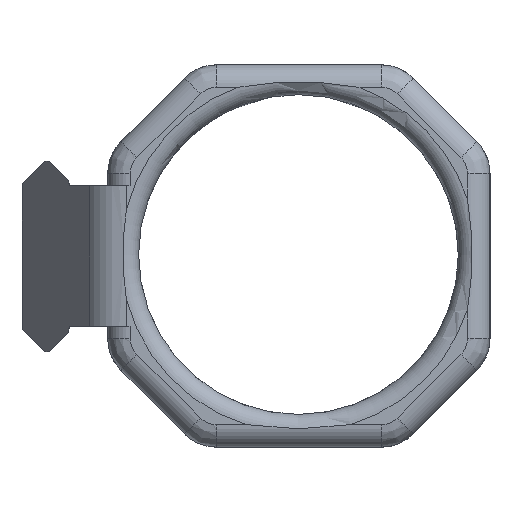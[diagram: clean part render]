
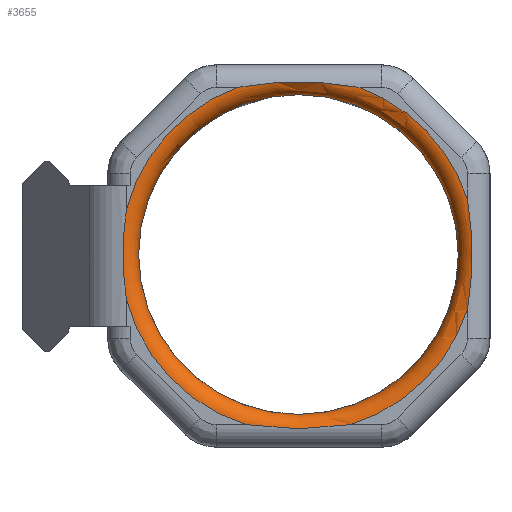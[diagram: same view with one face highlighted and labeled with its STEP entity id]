
A CAD part, left-side view. The second image highlights one B-rep face of the part: STEP entity #3655.
In plain terms, the highlighted toroidal (fillet/blend) face has major radius 19.771 mm and minor radius 2 mm.
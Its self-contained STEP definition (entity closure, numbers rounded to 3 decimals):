
#65=TOROIDAL_SURFACE('',#3895,19.771,2.);
#71=B_SPLINE_CURVE_WITH_KNOTS('',3,(#5442,#5443,#5444,#5445,#5446,#5447),
 .UNSPECIFIED.,.F.,.F.,(4,2,4),(0.498,0.996,0.998),
 .UNSPECIFIED.);
#72=B_SPLINE_CURVE_WITH_KNOTS('',3,(#5451,#5452,#5453,#5454,#5455,#5456,
#5457,#5458,#5459,#5460),.UNSPECIFIED.,.F.,.F.,(4,2,2,2,4),(-0.002,
0.,0.53,1.061,1.063),.UNSPECIFIED.);
#73=B_SPLINE_CURVE_WITH_KNOTS('',3,(#5464,#5465,#5466,#5467,#5468,#5469,
#5470,#5471,#5472,#5473),.UNSPECIFIED.,.F.,.F.,(4,2,2,2,4),(-0.002,
0.,0.584,1.169,1.171),.UNSPECIFIED.);
#74=B_SPLINE_CURVE_WITH_KNOTS('',3,(#5477,#5478,#5479,#5480,#5481,#5482,
#5483,#5484,#5485,#5486),.UNSPECIFIED.,.F.,.F.,(4,2,2,2,4),(-0.003,
0.,0.495,0.991,0.994),.UNSPECIFIED.);
#75=B_SPLINE_CURVE_WITH_KNOTS('',3,(#5489,#5490,#5491,#5492,#5493,#5494),
 .UNSPECIFIED.,.F.,.F.,(4,2,4),(-0.002,0.,0.498),
 .UNSPECIFIED.);
#286=FACE_OUTER_BOUND('',#485,.T.);
#485=EDGE_LOOP('',(#2614,#2615,#2616,#2617,#2618,#2619,#2620,#2621,#2622,
#2623,#2624,#2625,#2626));
#1461=CIRCLE('',#3896,17.771);
#1462=CIRCLE('',#3897,2.);
#1463=CIRCLE('',#3898,19.771);
#1464=CIRCLE('',#3899,19.771);
#1465=CIRCLE('',#3900,19.771);
#1466=CIRCLE('',#3901,19.771);
#1467=CIRCLE('',#3902,17.771);
#1619=VERTEX_POINT('',#5436);
#1620=VERTEX_POINT('',#5437);
#1621=VERTEX_POINT('',#5439);
#1622=VERTEX_POINT('',#5441);
#1623=VERTEX_POINT('',#5448);
#1624=VERTEX_POINT('',#5450);
#1625=VERTEX_POINT('',#5461);
#1626=VERTEX_POINT('',#5463);
#1627=VERTEX_POINT('',#5474);
#1628=VERTEX_POINT('',#5476);
#1629=VERTEX_POINT('',#5487);
#1999=EDGE_CURVE('',#1619,#1620,#1461,.T.);
#2000=EDGE_CURVE('',#1620,#1621,#1462,.T.);
#2001=EDGE_CURVE('',#1621,#1622,#71,.T.);
#2002=EDGE_CURVE('',#1622,#1623,#1463,.T.);
#2003=EDGE_CURVE('',#1623,#1624,#72,.T.);
#2004=EDGE_CURVE('',#1624,#1625,#1464,.T.);
#2005=EDGE_CURVE('',#1625,#1626,#73,.T.);
#2006=EDGE_CURVE('',#1626,#1627,#1465,.T.);
#2007=EDGE_CURVE('',#1627,#1628,#74,.T.);
#2008=EDGE_CURVE('',#1628,#1629,#1466,.T.);
#2009=EDGE_CURVE('',#1629,#1621,#75,.T.);
#2010=EDGE_CURVE('',#1620,#1619,#1467,.T.);
#2614=ORIENTED_EDGE('',*,*,#1999,.T.);
#2615=ORIENTED_EDGE('',*,*,#2000,.T.);
#2616=ORIENTED_EDGE('',*,*,#2001,.T.);
#2617=ORIENTED_EDGE('',*,*,#2002,.T.);
#2618=ORIENTED_EDGE('',*,*,#2003,.T.);
#2619=ORIENTED_EDGE('',*,*,#2004,.T.);
#2620=ORIENTED_EDGE('',*,*,#2005,.T.);
#2621=ORIENTED_EDGE('',*,*,#2006,.T.);
#2622=ORIENTED_EDGE('',*,*,#2007,.T.);
#2623=ORIENTED_EDGE('',*,*,#2008,.T.);
#2624=ORIENTED_EDGE('',*,*,#2009,.T.);
#2625=ORIENTED_EDGE('',*,*,#2000,.F.);
#2626=ORIENTED_EDGE('',*,*,#2010,.T.);
#3655=ADVANCED_FACE('',(#286),#65,.T.);
#3895=AXIS2_PLACEMENT_3D('',#5435,#4336,#4337);
#3896=AXIS2_PLACEMENT_3D('',#5438,#4338,#4339);
#3897=AXIS2_PLACEMENT_3D('',#5440,#4340,#4341);
#3898=AXIS2_PLACEMENT_3D('',#5449,#4342,#4343);
#3899=AXIS2_PLACEMENT_3D('',#5462,#4344,#4345);
#3900=AXIS2_PLACEMENT_3D('',#5475,#4346,#4347);
#3901=AXIS2_PLACEMENT_3D('',#5488,#4348,#4349);
#3902=AXIS2_PLACEMENT_3D('',#5495,#4350,#4351);
#4336=DIRECTION('center_axis',(-1.,0.,0.));
#4337=DIRECTION('ref_axis',(0.,0.,1.));
#4338=DIRECTION('center_axis',(1.,0.,0.));
#4339=DIRECTION('ref_axis',(0.,-1.,0.));
#4340=DIRECTION('center_axis',(0.,-1.,0.));
#4341=DIRECTION('ref_axis',(0.,0.,-1.));
#4342=DIRECTION('center_axis',(-1.,0.,0.));
#4343=DIRECTION('ref_axis',(0.,-1.,0.));
#4344=DIRECTION('center_axis',(-1.,0.,0.));
#4345=DIRECTION('ref_axis',(0.,-1.,0.));
#4346=DIRECTION('center_axis',(-1.,0.,0.));
#4347=DIRECTION('ref_axis',(0.,-1.,0.));
#4348=DIRECTION('center_axis',(-1.,0.,0.));
#4349=DIRECTION('ref_axis',(0.,-1.,0.));
#4350=DIRECTION('center_axis',(1.,0.,0.));
#4351=DIRECTION('ref_axis',(0.,-1.,0.));
#5435=CARTESIAN_POINT('Origin',(154.494,184.064,13.948));
#5436=CARTESIAN_POINT('',(154.494,201.835,13.948));
#5437=CARTESIAN_POINT('',(154.494,184.064,-3.823));
#5438=CARTESIAN_POINT('Origin',(154.494,184.064,13.948));
#5439=CARTESIAN_POINT('',(152.536,184.064,-5.416));
#5440=CARTESIAN_POINT('Origin',(154.494,184.064,-5.823));
#5441=CARTESIAN_POINT('',(152.494,178.29,-4.961));
#5442=CARTESIAN_POINT('Ctrl Pts',(152.536,184.064,-5.416));
#5443=CARTESIAN_POINT('Ctrl Pts',(152.536,181.868,-5.416));
#5444=CARTESIAN_POINT('Ctrl Pts',(152.494,179.949,-5.222));
#5445=CARTESIAN_POINT('Ctrl Pts',(152.494,178.302,-4.963));
#5446=CARTESIAN_POINT('Ctrl Pts',(152.494,178.296,-4.962));
#5447=CARTESIAN_POINT('Ctrl Pts',(152.494,178.29,-4.961));
#5448=CARTESIAN_POINT('',(152.494,165.268,7.813));
#5449=CARTESIAN_POINT('Origin',(152.494,184.064,13.948));
#5450=CARTESIAN_POINT('',(152.494,165.268,20.084));
#5451=CARTESIAN_POINT('Ctrl Pts',(152.494,165.268,7.813));
#5452=CARTESIAN_POINT('Ctrl Pts',(152.494,165.267,7.819));
#5453=CARTESIAN_POINT('Ctrl Pts',(152.494,165.266,7.825));
#5454=CARTESIAN_POINT('Ctrl Pts',(152.494,164.973,9.575));
#5455=CARTESIAN_POINT('Ctrl Pts',(152.548,164.753,11.615));
#5456=CARTESIAN_POINT('Ctrl Pts',(152.548,164.753,16.281));
#5457=CARTESIAN_POINT('Ctrl Pts',(152.494,164.973,18.321));
#5458=CARTESIAN_POINT('Ctrl Pts',(152.494,165.266,20.071));
#5459=CARTESIAN_POINT('Ctrl Pts',(152.494,165.267,20.078));
#5460=CARTESIAN_POINT('Ctrl Pts',(152.494,165.268,20.084));
#5461=CARTESIAN_POINT('',(152.494,177.334,32.539));
#5462=CARTESIAN_POINT('Origin',(152.494,184.064,13.948));
#5463=CARTESIAN_POINT('',(152.494,190.793,32.539));
#5464=CARTESIAN_POINT('Ctrl Pts',(152.494,177.334,32.539));
#5465=CARTESIAN_POINT('Ctrl Pts',(152.494,177.34,32.54));
#5466=CARTESIAN_POINT('Ctrl Pts',(152.494,177.346,32.541));
#5467=CARTESIAN_POINT('Ctrl Pts',(152.495,179.267,32.897));
#5468=CARTESIAN_POINT('Ctrl Pts',(152.573,181.505,33.163));
#5469=CARTESIAN_POINT('Ctrl Pts',(152.573,186.623,33.163));
#5470=CARTESIAN_POINT('Ctrl Pts',(152.495,188.86,32.897));
#5471=CARTESIAN_POINT('Ctrl Pts',(152.494,190.781,32.541));
#5472=CARTESIAN_POINT('Ctrl Pts',(152.494,190.787,32.54));
#5473=CARTESIAN_POINT('Ctrl Pts',(152.494,190.793,32.539));
#5474=CARTESIAN_POINT('',(152.494,203.198,18.924));
#5475=CARTESIAN_POINT('Origin',(152.494,184.064,13.948));
#5476=CARTESIAN_POINT('',(152.494,203.198,8.972));
#5477=CARTESIAN_POINT('Ctrl Pts',(152.494,203.198,18.924));
#5478=CARTESIAN_POINT('Ctrl Pts',(152.494,203.2,18.913));
#5479=CARTESIAN_POINT('Ctrl Pts',(152.494,203.202,18.903));
#5480=CARTESIAN_POINT('Ctrl Pts',(152.494,203.458,17.26));
#5481=CARTESIAN_POINT('Ctrl Pts',(152.509,203.588,15.612));
#5482=CARTESIAN_POINT('Ctrl Pts',(152.509,203.588,12.285));
#5483=CARTESIAN_POINT('Ctrl Pts',(152.494,203.458,10.636));
#5484=CARTESIAN_POINT('Ctrl Pts',(152.494,203.202,8.994));
#5485=CARTESIAN_POINT('Ctrl Pts',(152.494,203.2,8.983));
#5486=CARTESIAN_POINT('Ctrl Pts',(152.494,203.198,8.972));
#5487=CARTESIAN_POINT('',(152.494,189.837,-4.961));
#5488=CARTESIAN_POINT('Origin',(152.494,184.064,13.948));
#5489=CARTESIAN_POINT('Ctrl Pts',(152.494,189.837,-4.961));
#5490=CARTESIAN_POINT('Ctrl Pts',(152.494,189.831,-4.962));
#5491=CARTESIAN_POINT('Ctrl Pts',(152.494,189.825,-4.963));
#5492=CARTESIAN_POINT('Ctrl Pts',(152.494,188.178,-5.222));
#5493=CARTESIAN_POINT('Ctrl Pts',(152.536,186.259,-5.416));
#5494=CARTESIAN_POINT('Ctrl Pts',(152.536,184.064,-5.416));
#5495=CARTESIAN_POINT('Origin',(154.494,184.064,13.948));
